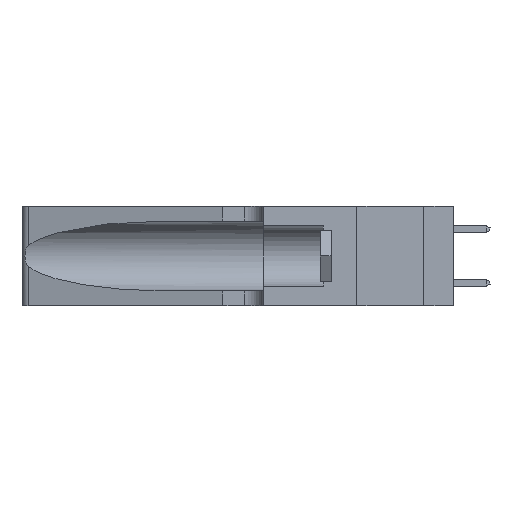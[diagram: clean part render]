
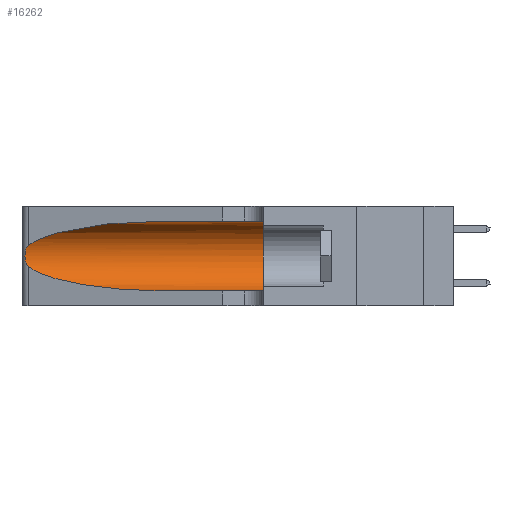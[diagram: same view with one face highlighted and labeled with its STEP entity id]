
A CAD part, left-side view. The second image highlights one B-rep face of the part: STEP entity #16262.
In plain terms, the highlighted cylindrical face has radius 3.308 mm (diameter 6.617 mm), a partial arc.
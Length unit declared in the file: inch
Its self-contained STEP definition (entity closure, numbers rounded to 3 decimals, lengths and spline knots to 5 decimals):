
#768 = VECTOR ( 'NONE', #41697, 39.37008 ) ;
#1048 = ORIENTED_EDGE ( 'NONE', *, *, #20536, .T. ) ;
#2294 = DIRECTION ( 'NONE',  ( 0., 0., -1. ) ) ;
#2610 = VECTOR ( 'NONE', #23817, 39.37008 ) ;
#5170 = CARTESIAN_POINT ( 'NONE',  ( 0.1305, 0.72297, 0.05475 ) ) ;
#7239 = EDGE_CURVE ( 'NONE', #20621, #30822, #15394, .T. ) ;
#7665 = CARTESIAN_POINT ( 'NONE',  ( 0.18966, 0.96281, 0.31525 ) ) ;
#8127 = VERTEX_POINT ( 'NONE', #40093 ) ;
#8881 = CARTESIAN_POINT ( 'NONE',  ( 0.25787, 1.23484, 0.2124 ) ) ;
#8986 = VERTEX_POINT ( 'NONE', #44631 ) ;
#10641 = CARTESIAN_POINT ( 'NONE',  ( 0.1305, 0.72297, 0.31525 ) ) ;
#12393 = EDGE_CURVE ( 'NONE', #29626, #20621, #44231, .T. ) ;
#12553 = CARTESIAN_POINT ( 'NONE',  ( 0.26017, 1.23833, 0.17102 ) ) ;
#13482 = EDGE_LOOP ( 'NONE', ( #22007, #32448, #29231, #1048, #17259, #46578 ) ) ;
#13585 = CIRCLE ( 'NONE', #43395, 0.13025 ) ;
#13842 = DIRECTION ( 'NONE',  ( 0., -1., 0. ) ) ;
#14370 = LINE ( 'NONE', #43678, #768 ) ;
#15394 = B_SPLINE_CURVE_WITH_KNOTS ( 'NONE', 3,
 ( #41934, #16658, #30699, #8881, #34324, #45718, #27674, #31309, #12553, #37991, #23841, #42868, #28140, #46182 ),
 .UNSPECIFIED., .F., .F.,
 ( 4, 2, 2, 2, 2, 2, 4 ),
 ( 0., 0.00027, 0.00053, 0.00107, 0.0016, 0.00187, 0.00214 ),
 .UNSPECIFIED. ) ;
#15489 = CARTESIAN_POINT ( 'NONE',  ( 0.25487, 1.22718, 0.14631 ) ) ;
#16204 = VERTEX_POINT ( 'NONE', #35297 ) ;
#16262 = ADVANCED_FACE ( 'NONE', ( #20068 ), #17228, .F. ) ;
#16281 = EDGE_CURVE ( 'NONE', #29626, #8986, #14370, .T. ) ;
#16658 = CARTESIAN_POINT ( 'NONE',  ( 0.25555, 1.22994, 0.2215 ) ) ;
#17228 = CYLINDRICAL_SURFACE ( 'NONE', #20207, 0.13025 ) ;
#17259 = ORIENTED_EDGE ( 'NONE', *, *, #25018, .F. ) ;
#18321 = CARTESIAN_POINT ( 'NONE',  ( 0.1305, 0.72297, 0.31525 ) ) ;
#20068 = FACE_OUTER_BOUND ( 'NONE', #13482, .T. ) ;
#20207 = AXIS2_PLACEMENT_3D ( 'NONE', #46390, #13842, #2294 ) ;
#20536 = EDGE_CURVE ( 'NONE', #16204, #8127, #38952, .T. ) ;
#20621 = VERTEX_POINT ( 'NONE', #31135 ) ;
#22007 = ORIENTED_EDGE ( 'NONE', *, *, #12393, .T. ) ;
#22221 = DIRECTION ( 'NONE',  ( 0., 0., 1. ) ) ;
#22280 = CARTESIAN_POINT ( 'NONE',  ( 0.25487, 1.22718, 0.22369 ) ) ;
#23817 = DIRECTION ( 'NONE',  ( 0., -1., 0. ) ) ;
#23841 = CARTESIAN_POINT ( 'NONE',  ( 0.25789, 1.23486, 0.15765 ) ) ;
#24048 = EDGE_CURVE ( 'NONE', #30822, #16204, #26510, .T. ) ;
#25018 = EDGE_CURVE ( 'NONE', #8986, #8127, #13585, .T. ) ;
#26510 =( BOUNDED_CURVE ( )  B_SPLINE_CURVE ( 3, ( #15489, #41521, #37285, #5170 ),
 .UNSPECIFIED., .F., .T. ) 
 B_SPLINE_CURVE_WITH_KNOTS ( ( 4, 4 ),
 ( 3.44316, 4.71239 ),
 .UNSPECIFIED. ) 
 CURVE ( )  GEOMETRIC_REPRESENTATION_ITEM ( )  RATIONAL_B_SPLINE_CURVE ( ( 1., 0.87, 0.87, 1. ) ) 
 REPRESENTATION_ITEM ( '' )  );
#27674 = CARTESIAN_POINT ( 'NONE',  ( 0.26075, 1.23896, 0.19203 ) ) ;
#28140 = CARTESIAN_POINT ( 'NONE',  ( 0.25555, 1.22993, 0.14849 ) ) ;
#29231 = ORIENTED_EDGE ( 'NONE', *, *, #24048, .T. ) ;
#29626 = VERTEX_POINT ( 'NONE', #10641 ) ;
#30699 = CARTESIAN_POINT ( 'NONE',  ( 0.25639, 1.23184, 0.21858 ) ) ;
#30822 = VERTEX_POINT ( 'NONE', #45939 ) ;
#31135 = CARTESIAN_POINT ( 'NONE',  ( 0.25487, 1.22718, 0.22369 ) ) ;
#31309 = CARTESIAN_POINT ( 'NONE',  ( 0.26075, 1.23896, 0.178 ) ) ;
#32448 = ORIENTED_EDGE ( 'NONE', *, *, #7239, .T. ) ;
#34324 = CARTESIAN_POINT ( 'NONE',  ( 0.25854, 1.2359, 0.20912 ) ) ;
#35297 = CARTESIAN_POINT ( 'NONE',  ( 0.1305, 0.72297, 0.05475 ) ) ;
#36546 = DIRECTION ( 'NONE',  ( 0., 1., 0. ) ) ;
#36765 = CARTESIAN_POINT ( 'NONE',  ( 0.2373, 1.15595, 0.28018 ) ) ;
#37285 = CARTESIAN_POINT ( 'NONE',  ( 0.18966, 0.96281, 0.05475 ) ) ;
#37991 = CARTESIAN_POINT ( 'NONE',  ( 0.25856, 1.23593, 0.16098 ) ) ;
#38952 = LINE ( 'NONE', #42525, #2610 ) ;
#39731 = CARTESIAN_POINT ( 'NONE',  ( 0.1305, 0.35, 0.185 ) ) ;
#40093 = CARTESIAN_POINT ( 'NONE',  ( 0.1305, 0.35, 0.05475 ) ) ;
#41521 = CARTESIAN_POINT ( 'NONE',  ( 0.2373, 1.15595, 0.08982 ) ) ;
#41697 = DIRECTION ( 'NONE',  ( 0., -1., 0. ) ) ;
#41934 = CARTESIAN_POINT ( 'NONE',  ( 0.25487, 1.22718, 0.22369 ) ) ;
#42525 = CARTESIAN_POINT ( 'NONE',  ( 0.1305, 1.61858, 0.05475 ) ) ;
#42868 = CARTESIAN_POINT ( 'NONE',  ( 0.25639, 1.23186, 0.15144 ) ) ;
#43395 = AXIS2_PLACEMENT_3D ( 'NONE', #39731, #36546, #22221 ) ;
#43678 = CARTESIAN_POINT ( 'NONE',  ( 0.1305, 1.61858, 0.31525 ) ) ;
#44231 =( BOUNDED_CURVE ( )  B_SPLINE_CURVE ( 3, ( #18321, #7665, #36765, #22280 ),
 .UNSPECIFIED., .F., .T. ) 
 B_SPLINE_CURVE_WITH_KNOTS ( ( 4, 4 ),
 ( 1.5708, 2.84003 ),
 .UNSPECIFIED. ) 
 CURVE ( )  GEOMETRIC_REPRESENTATION_ITEM ( )  RATIONAL_B_SPLINE_CURVE ( ( 1., 0.87, 0.87, 1. ) ) 
 REPRESENTATION_ITEM ( '' )  );
#44631 = CARTESIAN_POINT ( 'NONE',  ( 0.1305, 0.35, 0.31525 ) ) ;
#45718 = CARTESIAN_POINT ( 'NONE',  ( 0.26018, 1.23835, 0.19895 ) ) ;
#45939 = CARTESIAN_POINT ( 'NONE',  ( 0.25487, 1.22718, 0.14631 ) ) ;
#46182 = CARTESIAN_POINT ( 'NONE',  ( 0.25487, 1.22718, 0.14631 ) ) ;
#46390 = CARTESIAN_POINT ( 'NONE',  ( 0.1305, 1.61858, 0.185 ) ) ;
#46578 = ORIENTED_EDGE ( 'NONE', *, *, #16281, .F. ) ;
